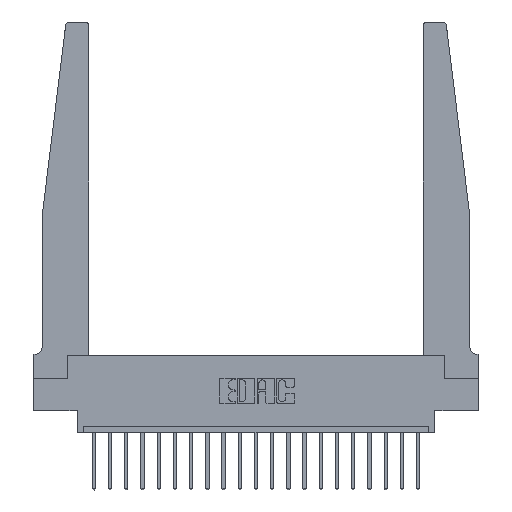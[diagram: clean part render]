
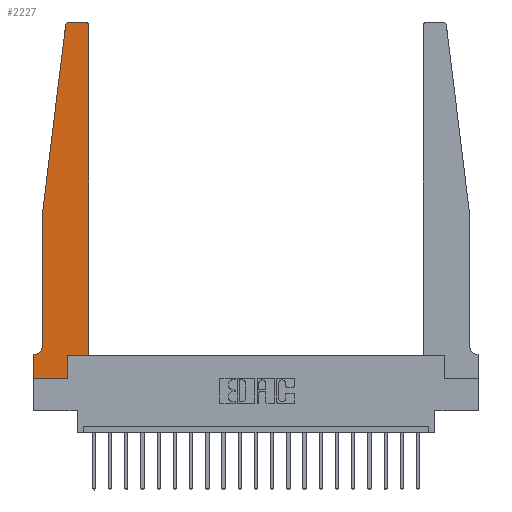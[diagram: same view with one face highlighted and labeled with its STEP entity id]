
A CAD part, top view. The second image highlights one B-rep face of the part: STEP entity #2227.
In plain terms, the highlighted planar face has unit normal (0, 0, 1).
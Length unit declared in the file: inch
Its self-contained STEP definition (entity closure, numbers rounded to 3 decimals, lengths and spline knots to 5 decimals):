
#141 = CARTESIAN_POINT ( 'NONE',  ( 0., 0.1875, 0.37 ) ) ;
#211 = EDGE_CURVE ( 'NONE', #17754, #11265, #5118, .T. ) ;
#289 = DIRECTION ( 'NONE',  ( 0., 1., 0. ) ) ;
#885 = EDGE_CURVE ( 'NONE', #3978, #3849, #15887, .T. ) ;
#933 = ORIENTED_EDGE ( 'NONE', *, *, #18656, .T. ) ;
#1102 = EDGE_CURVE ( 'NONE', #9527, #20496, #14645, .T. ) ;
#1183 = DIRECTION ( 'NONE',  ( 0., -1., 0. ) ) ;
#1460 = LINE ( 'NONE', #11502, #17491 ) ;
#1828 = DIRECTION ( 'NONE',  ( 0., 0., 1. ) ) ;
#1932 = DIRECTION ( 'NONE',  ( -1., 0., 0. ) ) ;
#1970 = ORIENTED_EDGE ( 'NONE', *, *, #885, .T. ) ;
#2227 = ADVANCED_FACE ( 'NONE', ( #17099 ), #9546, .T. ) ;
#3020 = EDGE_CURVE ( 'NONE', #11265, #4267, #3753, .T. ) ;
#3113 = CARTESIAN_POINT ( 'NONE',  ( 0.27653, 2.72, 0.37 ) ) ;
#3169 = CARTESIAN_POINT ( 'NONE',  ( 0.425, 0.18, 0.37 ) ) ;
#3735 = EDGE_LOOP ( 'NONE', ( #19467, #8204, #11337, #17506, #1970, #13883, #19786, #4480, #7416, #933, #13409, #9465 ) ) ;
#3753 = LINE ( 'NONE', #10219, #11538 ) ;
#3765 = CARTESIAN_POINT ( 'NONE',  ( 0., 0., 0.37 ) ) ;
#3849 = VERTEX_POINT ( 'NONE', #15929 ) ;
#3978 = VERTEX_POINT ( 'NONE', #9968 ) ;
#4112 = DIRECTION ( 'NONE',  ( 0., -1., 0. ) ) ;
#4267 = VERTEX_POINT ( 'NONE', #7827 ) ;
#4480 = ORIENTED_EDGE ( 'NONE', *, *, #8813, .T. ) ;
#4724 = DIRECTION ( 'NONE',  ( 0., 0., 1. ) ) ;
#4966 = CARTESIAN_POINT ( 'NONE',  ( 0.425, 2.72, 0.37 ) ) ;
#4987 = DIRECTION ( 'NONE',  ( 1., 0., 0. ) ) ;
#5118 = CIRCLE ( 'NONE', #14066, 0.03 ) ;
#5310 = EDGE_CURVE ( 'NONE', #12042, #13895, #7783, .T. ) ;
#5686 = VERTEX_POINT ( 'NONE', #9959 ) ;
#5743 = EDGE_CURVE ( 'NONE', #13895, #7630, #13577, .T. ) ;
#6131 = CARTESIAN_POINT ( 'NONE',  ( 0.24675, 2.72367, 0.37 ) ) ;
#6374 = CARTESIAN_POINT ( 'NONE',  ( 0.2605, 0.18, 0.37 ) ) ;
#7049 = VECTOR ( 'NONE', #1183, 39.37008 ) ;
#7256 = CARTESIAN_POINT ( 'NONE',  ( 0., 0., 0.37 ) ) ;
#7416 = ORIENTED_EDGE ( 'NONE', *, *, #13109, .T. ) ;
#7630 = VERTEX_POINT ( 'NONE', #18646 ) ;
#7783 = LINE ( 'NONE', #9123, #15323 ) ;
#7827 = CARTESIAN_POINT ( 'NONE',  ( 0.065, 1.25, 0.37 ) ) ;
#7963 = EDGE_CURVE ( 'NONE', #7630, #17754, #17722, .T. ) ;
#8095 = LINE ( 'NONE', #14463, #17400 ) ;
#8204 = ORIENTED_EDGE ( 'NONE', *, *, #211, .T. ) ;
#8379 = DIRECTION ( 'NONE',  ( -0.122, -0.992, 0. ) ) ;
#8547 = CARTESIAN_POINT ( 'NONE',  ( 0.395, 2.72, 0.37 ) ) ;
#8813 = EDGE_CURVE ( 'NONE', #20496, #11467, #9686, .T. ) ;
#8968 = VECTOR ( 'NONE', #289, 39.37008 ) ;
#8971 = CARTESIAN_POINT ( 'NONE',  ( 0.065, 1.25, 0.37 ) ) ;
#9123 = CARTESIAN_POINT ( 'NONE',  ( 0.425, 0.18, 0.37 ) ) ;
#9465 = ORIENTED_EDGE ( 'NONE', *, *, #5743, .T. ) ;
#9527 = VERTEX_POINT ( 'NONE', #20258 ) ;
#9546 = PLANE ( 'NONE',  #17702 ) ;
#9551 = DIRECTION ( 'NONE',  ( 1., 0., 0. ) ) ;
#9686 = LINE ( 'NONE', #16626, #19750 ) ;
#9866 = VECTOR ( 'NONE', #4112, 39.37008 ) ;
#9959 = CARTESIAN_POINT ( 'NONE',  ( 0.2605, 0.18, 0.37 ) ) ;
#9968 = CARTESIAN_POINT ( 'NONE',  ( 0.065, 0.2375, 0.37 ) ) ;
#10137 = CARTESIAN_POINT ( 'NONE',  ( 0.2605, 0., 0.37 ) ) ;
#10219 = CARTESIAN_POINT ( 'NONE',  ( 0.065, 1.25, 0.37 ) ) ;
#11155 = DIRECTION ( 'NONE',  ( 0., 0., -1. ) ) ;
#11230 = DIRECTION ( 'NONE',  ( -1., 0., 0. ) ) ;
#11265 = VERTEX_POINT ( 'NONE', #6131 ) ;
#11337 = ORIENTED_EDGE ( 'NONE', *, *, #3020, .T. ) ;
#11424 = DIRECTION ( 'NONE',  ( -1., 0., 0. ) ) ;
#11467 = VERTEX_POINT ( 'NONE', #10137 ) ;
#11502 = CARTESIAN_POINT ( 'NONE',  ( 0.065, 0.1875, 0.37 ) ) ;
#11538 = VECTOR ( 'NONE', #8379, 39.37008 ) ;
#12042 = VERTEX_POINT ( 'NONE', #3169 ) ;
#12110 = AXIS2_PLACEMENT_3D ( 'NONE', #8547, #14932, #18165 ) ;
#13109 = EDGE_CURVE ( 'NONE', #11467, #5686, #18528, .T. ) ;
#13242 = CARTESIAN_POINT ( 'NONE',  ( 0.25, 2.75, 0.37 ) ) ;
#13409 = ORIENTED_EDGE ( 'NONE', *, *, #5310, .T. ) ;
#13471 = VECTOR ( 'NONE', #1932, 39.37008 ) ;
#13577 = CIRCLE ( 'NONE', #12110, 0.03 ) ;
#13782 = EDGE_CURVE ( 'NONE', #3849, #9527, #1460, .T. ) ;
#13883 = ORIENTED_EDGE ( 'NONE', *, *, #13782, .T. ) ;
#13895 = VERTEX_POINT ( 'NONE', #4966 ) ;
#14066 = AXIS2_PLACEMENT_3D ( 'NONE', #3113, #4724, #14409 ) ;
#14409 = DIRECTION ( 'NONE',  ( 1., 0., 0. ) ) ;
#14463 = CARTESIAN_POINT ( 'NONE',  ( 0.425, 0.18, 0.37 ) ) ;
#14645 = LINE ( 'NONE', #7256, #9866 ) ;
#14932 = DIRECTION ( 'NONE',  ( 0., 0., 1. ) ) ;
#15323 = VECTOR ( 'NONE', #15424, 39.37008 ) ;
#15424 = DIRECTION ( 'NONE',  ( 0., 1., 0. ) ) ;
#15887 = CIRCLE ( 'NONE', #16065, 0.05 ) ;
#15929 = CARTESIAN_POINT ( 'NONE',  ( 0.015, 0.1875, 0.37 ) ) ;
#16065 = AXIS2_PLACEMENT_3D ( 'NONE', #20761, #11155, #11230 ) ;
#16626 = CARTESIAN_POINT ( 'NONE',  ( 0., 0., 0.37 ) ) ;
#17099 = FACE_OUTER_BOUND ( 'NONE', #3735, .T. ) ;
#17232 = EDGE_CURVE ( 'NONE', #4267, #3978, #17877, .T. ) ;
#17400 = VECTOR ( 'NONE', #9551, 39.37008 ) ;
#17491 = VECTOR ( 'NONE', #11424, 39.37008 ) ;
#17506 = ORIENTED_EDGE ( 'NONE', *, *, #17232, .T. ) ;
#17702 = AXIS2_PLACEMENT_3D ( 'NONE', #141, #1828, #4987 ) ;
#17722 = LINE ( 'NONE', #13242, #13471 ) ;
#17754 = VERTEX_POINT ( 'NONE', #20186 ) ;
#17877 = LINE ( 'NONE', #8971, #7049 ) ;
#18043 = DIRECTION ( 'NONE',  ( 1., 0., 0. ) ) ;
#18165 = DIRECTION ( 'NONE',  ( 1., 0., 0. ) ) ;
#18528 = LINE ( 'NONE', #6374, #8968 ) ;
#18646 = CARTESIAN_POINT ( 'NONE',  ( 0.395, 2.75, 0.37 ) ) ;
#18656 = EDGE_CURVE ( 'NONE', #5686, #12042, #8095, .T. ) ;
#19467 = ORIENTED_EDGE ( 'NONE', *, *, #7963, .T. ) ;
#19750 = VECTOR ( 'NONE', #18043, 39.37008 ) ;
#19786 = ORIENTED_EDGE ( 'NONE', *, *, #1102, .T. ) ;
#20186 = CARTESIAN_POINT ( 'NONE',  ( 0.27653, 2.75, 0.37 ) ) ;
#20258 = CARTESIAN_POINT ( 'NONE',  ( 0., 0.1875, 0.37 ) ) ;
#20496 = VERTEX_POINT ( 'NONE', #3765 ) ;
#20761 = CARTESIAN_POINT ( 'NONE',  ( 0.015, 0.2375, 0.37 ) ) ;
